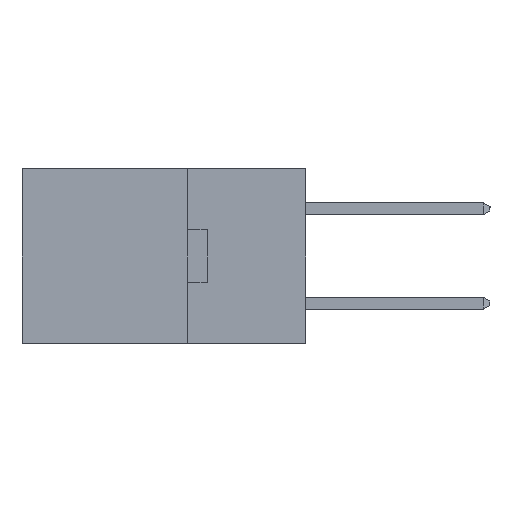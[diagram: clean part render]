
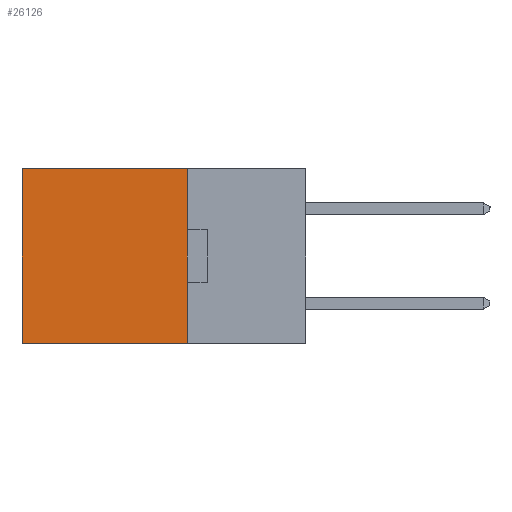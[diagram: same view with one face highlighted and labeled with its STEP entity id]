
A CAD part, left-side view. The second image highlights one B-rep face of the part: STEP entity #26126.
In plain terms, the highlighted planar face has unit normal (-1, 0, 0).
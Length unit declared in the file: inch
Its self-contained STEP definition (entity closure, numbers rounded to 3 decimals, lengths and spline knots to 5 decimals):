
#203 = VERTEX_POINT ( 'NONE', #24498 ) ;
#524 = CARTESIAN_POINT ( 'NONE',  ( 0.2615, 0.6, 0. ) ) ;
#944 = VECTOR ( 'NONE', #18793, 39.37008 ) ;
#2984 = DIRECTION ( 'NONE',  ( 0., 1., 0. ) ) ;
#3048 = DIRECTION ( 'NONE',  ( 0., 0., -1. ) ) ;
#6322 = VECTOR ( 'NONE', #22257, 39.37008 ) ;
#6913 = CARTESIAN_POINT ( 'NONE',  ( 0.2615, 0.25, -0.37 ) ) ;
#7531 = CARTESIAN_POINT ( 'NONE',  ( 0.2615, 0.6, -0.37 ) ) ;
#8752 = EDGE_CURVE ( 'NONE', #11774, #203, #20980, .T. ) ;
#8938 = LINE ( 'NONE', #6913, #6322 ) ;
#11774 = VERTEX_POINT ( 'NONE', #524 ) ;
#11811 = EDGE_CURVE ( 'NONE', #13207, #203, #25143, .T. ) ;
#12682 = DIRECTION ( 'NONE',  ( 0., 1., 0. ) ) ;
#13117 = VECTOR ( 'NONE', #2984, 39.37008 ) ;
#13207 = VERTEX_POINT ( 'NONE', #27490 ) ;
#13948 = PLANE ( 'NONE',  #23220 ) ;
#15184 = ORIENTED_EDGE ( 'NONE', *, *, #17736, .T. ) ;
#17736 = EDGE_CURVE ( 'NONE', #26872, #11774, #19269, .T. ) ;
#18051 = CARTESIAN_POINT ( 'NONE',  ( 0.2615, 0.25, -0.37 ) ) ;
#18793 = DIRECTION ( 'NONE',  ( 0., 0., -1. ) ) ;
#19048 = ORIENTED_EDGE ( 'NONE', *, *, #11811, .F. ) ;
#19269 = LINE ( 'NONE', #28174, #28205 ) ;
#20980 = LINE ( 'NONE', #7531, #944 ) ;
#22257 = DIRECTION ( 'NONE',  ( 0., 0., -1. ) ) ;
#22586 = DIRECTION ( 'NONE',  ( 1., 0., 0. ) ) ;
#22850 = EDGE_CURVE ( 'NONE', #26872, #13207, #8938, .T. ) ;
#23220 = AXIS2_PLACEMENT_3D ( 'NONE', #18051, #22586, #3048 ) ;
#23373 = ORIENTED_EDGE ( 'NONE', *, *, #22850, .F. ) ;
#24498 = CARTESIAN_POINT ( 'NONE',  ( 0.2615, 0.6, -0.37 ) ) ;
#25143 = LINE ( 'NONE', #27330, #13117 ) ;
#25189 = EDGE_LOOP ( 'NONE', ( #27307, #19048, #23373, #15184 ) ) ;
#26126 = ADVANCED_FACE ( 'NONE', ( #27398 ), #13948, .F. ) ;
#26872 = VERTEX_POINT ( 'NONE', #28218 ) ;
#27307 = ORIENTED_EDGE ( 'NONE', *, *, #8752, .T. ) ;
#27330 = CARTESIAN_POINT ( 'NONE',  ( 0.2615, 0.25, -0.37 ) ) ;
#27398 = FACE_OUTER_BOUND ( 'NONE', #25189, .T. ) ;
#27490 = CARTESIAN_POINT ( 'NONE',  ( 0.2615, 0.25, -0.37 ) ) ;
#28174 = CARTESIAN_POINT ( 'NONE',  ( 0.2615, 0.25, 0. ) ) ;
#28205 = VECTOR ( 'NONE', #12682, 39.37008 ) ;
#28218 = CARTESIAN_POINT ( 'NONE',  ( 0.2615, 0.25, 0. ) ) ;
